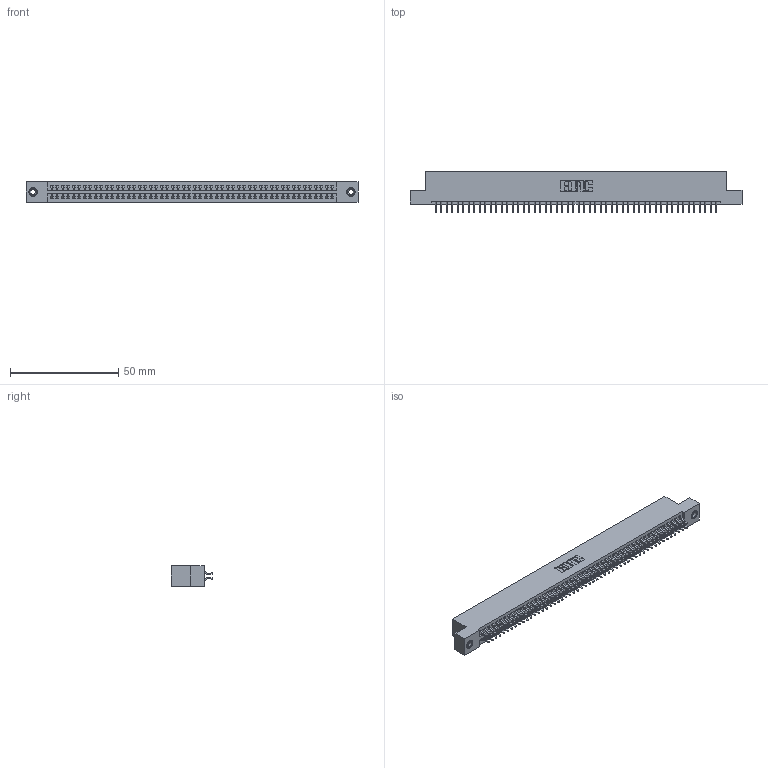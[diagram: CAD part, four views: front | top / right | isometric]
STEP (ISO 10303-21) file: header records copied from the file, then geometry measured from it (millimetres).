
FILE_DESCRIPTION (( 'STEP AP203' ), '1' );
FILE_NAME ('395-104-556-208.STEP', '2019-10-26T21:55:08', ( '' ), ( '' ), 'SwSTEP 2.0', 'SolidWorks 2016', '' );
FILE_SCHEMA (( 'CONFIG_CONTROL_DESIGN' ));
Length unit declared in the file: inch
Products named in the file (4): 395-104-556-208; 345 Part_Flush Mounting Lugs - 0.156 Dia-TI; 345-292-001_556 Tail; 345-250-001_345-250-003-102
Assembly tree (107 placements, depth 2):
  395-104-556-208
    345 Part_Flush Mounting Lugs - 0.156 Dia-TI
    345-292-001_556 Tail  x104
    345-250-001_345-250-003-102  x2
Bounding box: 153.29 x 19.24 x 9.4 mm (x, y, z)
Volume: 14972.8 mm3; surface area: 22248.4 mm2
Topology: 107 solids, 107 shells, 6010 faces, 17845 edges, 11750 vertices
Faces by surface type: plane 3960, cylinder 2034, cone 12, torus 4
Entity records: 40860 total; most frequent: CARTESIAN_POINT 6835, ORIENTED_EDGE 6750, DIRECTION 6029, EDGE_CURVE 3375, LINE 3007, VECTOR 3007, VERTEX_POINT 2244, AXIS2_PLACEMENT_3D 1511
